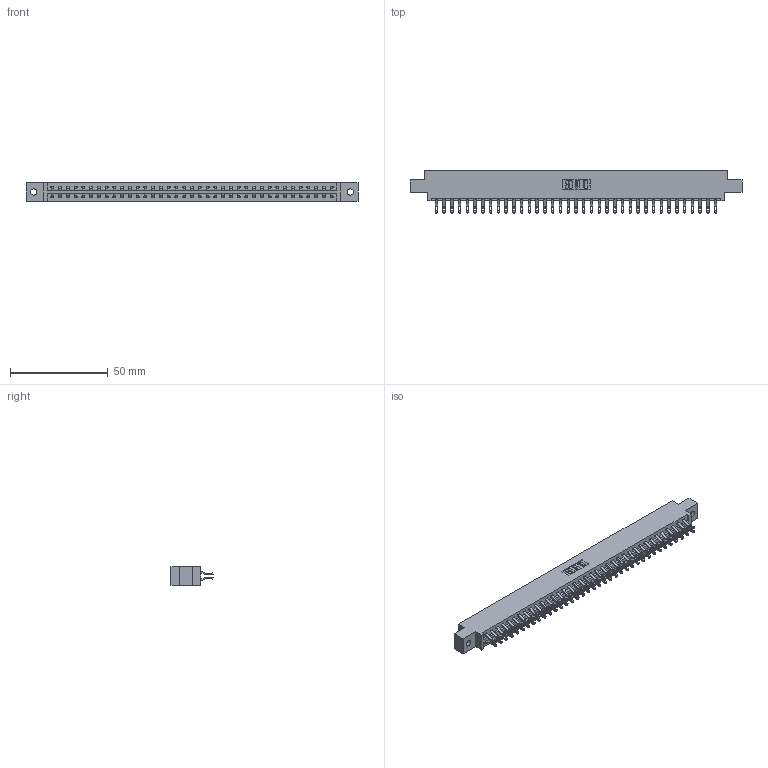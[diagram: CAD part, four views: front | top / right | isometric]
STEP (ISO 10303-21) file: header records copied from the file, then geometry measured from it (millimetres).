
FILE_DESCRIPTION (( 'STEP AP203' ), '1' );
FILE_NAME ('387-074-555-802.STEP', '2019-10-22T02:12:27', ( '' ), ( '' ), 'SwSTEP 2.0', 'SolidWorks 2016', '' );
FILE_SCHEMA (( 'CONFIG_CONTROL_DESIGN' ));
Length unit declared in the file: inch
Products named in the file (3): 337 Part_0.170 Offset - 0.128 Dia; 345-292-001_555 Tail; 387-074-555-802
Assembly tree (75 placements, depth 2):
  387-074-555-802
    337 Part_0.170 Offset - 0.128 Dia
    345-292-001_555 Tail  x74
Bounding box: 169.62 x 21.47 x 9.4 mm (x, y, z)
Volume: 17869.9 mm3; surface area: 20797.4 mm2
Topology: 75 solids, 75 shells, 4558 faces, 14309 edges, 9538 vertices
Faces by surface type: plane 2738, cylinder 1820
Entity records: 29795 total; most frequent: CARTESIAN_POINT 5060, ORIENTED_EDGE 4966, DIRECTION 4283, EDGE_CURVE 2483, VECTOR 2335, LINE 2335, VERTEX_POINT 1654, AXIS2_PLACEMENT_3D 974
